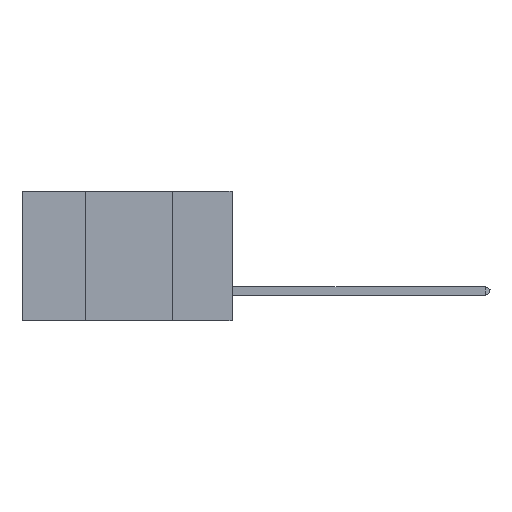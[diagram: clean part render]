
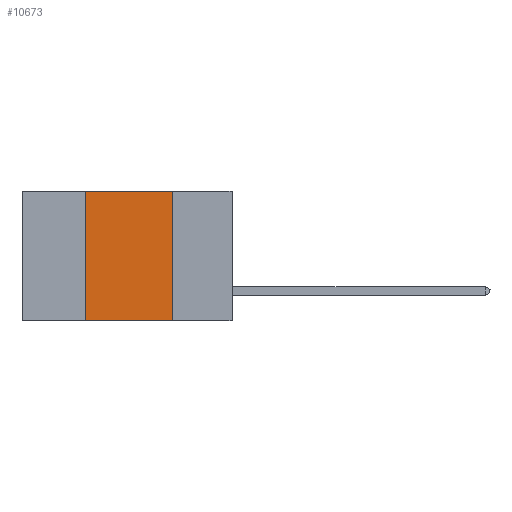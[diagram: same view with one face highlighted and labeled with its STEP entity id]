
A CAD part, left-side view. The second image highlights one B-rep face of the part: STEP entity #10673.
In plain terms, the highlighted planar face has unit normal (-1, 0, 0).
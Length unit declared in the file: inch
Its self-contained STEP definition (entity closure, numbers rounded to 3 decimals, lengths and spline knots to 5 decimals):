
#542 = VERTEX_POINT ( 'NONE', #11160 ) ;
#927 = DIRECTION ( 'NONE',  ( 1., 0., 0. ) ) ;
#928 = VECTOR ( 'NONE', #4165, 39.37008 ) ;
#1782 = CARTESIAN_POINT ( 'NONE',  ( 0., 0.17, 0. ) ) ;
#2047 = VECTOR ( 'NONE', #9016, 39.37008 ) ;
#3318 = VECTOR ( 'NONE', #8447, 39.37008 ) ;
#3739 = CARTESIAN_POINT ( 'NONE',  ( 0., 0.42, 0. ) ) ;
#3906 = DIRECTION ( 'NONE',  ( 0., -1., 0. ) ) ;
#4165 = DIRECTION ( 'NONE',  ( 0., -1., 0. ) ) ;
#4681 = LINE ( 'NONE', #10945, #17193 ) ;
#5196 = EDGE_CURVE ( 'NONE', #542, #12560, #10087, .T. ) ;
#8246 = ORIENTED_EDGE ( 'NONE', *, *, #10123, .F. ) ;
#8293 = EDGE_LOOP ( 'NONE', ( #10501, #8246, #9173, #13953 ) ) ;
#8447 = DIRECTION ( 'NONE',  ( 0., 0., 1. ) ) ;
#9016 = DIRECTION ( 'NONE',  ( 0., 0., -1. ) ) ;
#9098 = AXIS2_PLACEMENT_3D ( 'NONE', #18052, #927, #9627 ) ;
#9173 = ORIENTED_EDGE ( 'NONE', *, *, #13876, .F. ) ;
#9627 = DIRECTION ( 'NONE',  ( 0., 0., -1. ) ) ;
#9995 = CARTESIAN_POINT ( 'NONE',  ( 0., 0.17, -0.37 ) ) ;
#10087 = LINE ( 'NONE', #1782, #2047 ) ;
#10123 = EDGE_CURVE ( 'NONE', #15423, #542, #4681, .T. ) ;
#10501 = ORIENTED_EDGE ( 'NONE', *, *, #5196, .F. ) ;
#10673 = ADVANCED_FACE ( 'NONE', ( #16939 ), #16593, .F. ) ;
#10945 = CARTESIAN_POINT ( 'NONE',  ( 0., 0.6, 0. ) ) ;
#11160 = CARTESIAN_POINT ( 'NONE',  ( 0., 0.17, 0. ) ) ;
#11789 = LINE ( 'NONE', #3739, #3318 ) ;
#12078 = LINE ( 'NONE', #12400, #928 ) ;
#12196 = EDGE_CURVE ( 'NONE', #14063, #12560, #12078, .T. ) ;
#12400 = CARTESIAN_POINT ( 'NONE',  ( 0., 0.6, -0.37 ) ) ;
#12560 = VERTEX_POINT ( 'NONE', #9995 ) ;
#13140 = CARTESIAN_POINT ( 'NONE',  ( 0., 0.42, 0. ) ) ;
#13876 = EDGE_CURVE ( 'NONE', #14063, #15423, #11789, .T. ) ;
#13953 = ORIENTED_EDGE ( 'NONE', *, *, #12196, .T. ) ;
#14063 = VERTEX_POINT ( 'NONE', #17141 ) ;
#15423 = VERTEX_POINT ( 'NONE', #13140 ) ;
#16593 = PLANE ( 'NONE',  #9098 ) ;
#16939 = FACE_OUTER_BOUND ( 'NONE', #8293, .T. ) ;
#17141 = CARTESIAN_POINT ( 'NONE',  ( 0., 0.42, -0.37 ) ) ;
#17193 = VECTOR ( 'NONE', #3906, 39.37008 ) ;
#18052 = CARTESIAN_POINT ( 'NONE',  ( 0., 0.6, 0. ) ) ;
